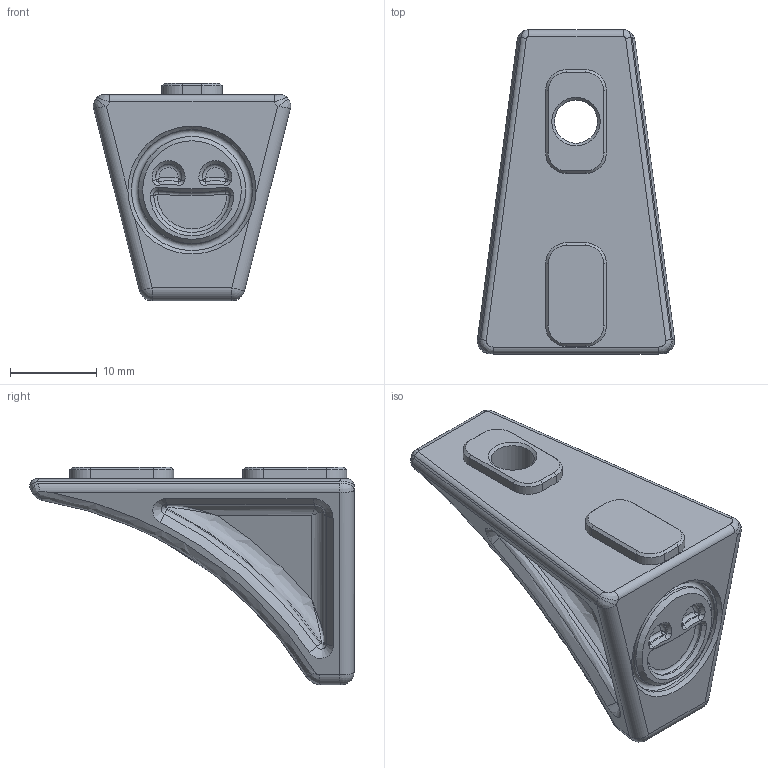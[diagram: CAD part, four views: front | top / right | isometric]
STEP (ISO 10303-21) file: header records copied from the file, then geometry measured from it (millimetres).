
FILE_DESCRIPTION(/* description */ (''),/* implementation_level */ '2;1');
FILE_NAME(/* name */ 'Laffs.step',/* time_stamp */ '2021-06-02T00:24:20-04:00',/* author */ (''),/* organization */ (''),/* preprocessor_version */ 'ST-DEVELOPER v18.1',/* originating_system */ 'Autodesk Translation Framework v10.9.0.1377',/* authorisation */ '');
FILE_SCHEMA (('AUTOMOTIVE_DESIGN { 1 0 10303 214 3 1 1 }'));
Length unit declared in the file: millimetre
Products named in the file (1): Laffs
Bounding box: 22.81 x 37.48 x 25.15 mm (x, y, z)
Volume: 5778.1 mm3; surface area: 3016.7 mm2
Topology: 1 solids, 1 shells, 177 faces, 400 edges, 219 vertices
Faces by surface type: cylinder 50, bspline 50, plane 41, cone 25, torus 9, sphere 2
Full cylindrical faces by diameter (mm): 5 x1, 9.3 x1, 12.4 x1, 14 x1
Entity records: 6596 total; most frequent: CARTESIAN_POINT 2894, ORIENTED_EDGE 772, DIRECTION 728, EDGE_CURVE 386, AXIS2_PLACEMENT_3D 287, VERTEX_POINT 219, EDGE_LOOP 187, FACE_OUTER_BOUND 177
